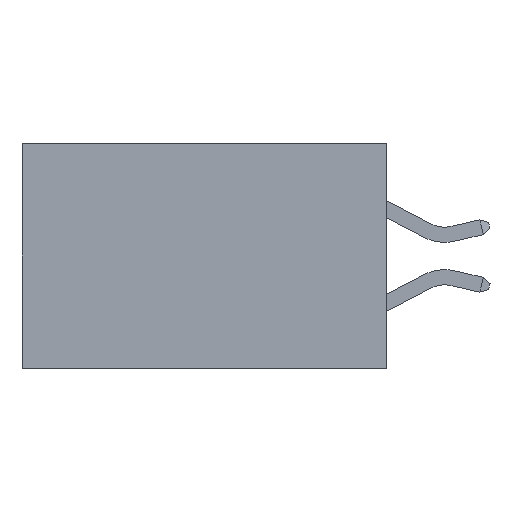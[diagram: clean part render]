
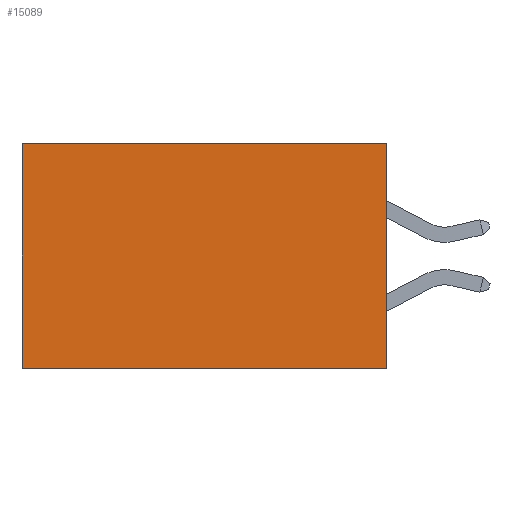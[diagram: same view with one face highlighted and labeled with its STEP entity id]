
A CAD part, left-side view. The second image highlights one B-rep face of the part: STEP entity #15089.
In plain terms, the highlighted planar face has unit normal (-1, 0, 0).
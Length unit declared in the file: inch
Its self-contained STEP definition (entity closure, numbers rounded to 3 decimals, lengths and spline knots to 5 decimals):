
#52 = VECTOR ( 'NONE', #13394, 39.37008 ) ;
#199 = LINE ( 'NONE', #14924, #10874 ) ;
#1112 = DIRECTION ( 'NONE',  ( 0., 0., -1. ) ) ;
#1361 = VECTOR ( 'NONE', #12651, 39.37008 ) ;
#1576 = CARTESIAN_POINT ( 'NONE',  ( 0.298, 0., 0. ) ) ;
#1749 = ORIENTED_EDGE ( 'NONE', *, *, #4311, .F. ) ;
#1804 = LINE ( 'NONE', #1576, #1361 ) ;
#1868 = EDGE_LOOP ( 'NONE', ( #5318, #17634, #1749, #15036 ) ) ;
#2588 = EDGE_CURVE ( 'NONE', #6344, #4546, #7381, .T. ) ;
#3395 = EDGE_CURVE ( 'NONE', #5895, #10210, #1804, .T. ) ;
#3590 = CARTESIAN_POINT ( 'NONE',  ( 0.298, 0., 0. ) ) ;
#3687 = LINE ( 'NONE', #9268, #52 ) ;
#3765 = CARTESIAN_POINT ( 'NONE',  ( 0.298, 0., 0. ) ) ;
#4311 = EDGE_CURVE ( 'NONE', #5895, #6344, #3687, .T. ) ;
#4328 = FACE_OUTER_BOUND ( 'NONE', #1868, .T. ) ;
#4546 = VERTEX_POINT ( 'NONE', #12288 ) ;
#5318 = ORIENTED_EDGE ( 'NONE', *, *, #7977, .T. ) ;
#5843 = CARTESIAN_POINT ( 'NONE',  ( 0.298, 0.6, 0. ) ) ;
#5895 = VERTEX_POINT ( 'NONE', #3590 ) ;
#6344 = VERTEX_POINT ( 'NONE', #8497 ) ;
#7381 = LINE ( 'NONE', #15487, #14379 ) ;
#7475 = DIRECTION ( 'NONE',  ( 0., 1., 0. ) ) ;
#7977 = EDGE_CURVE ( 'NONE', #10210, #4546, #199, .T. ) ;
#8098 = DIRECTION ( 'NONE',  ( 0., 0., -1. ) ) ;
#8497 = CARTESIAN_POINT ( 'NONE',  ( 0.298, 0., -0.37 ) ) ;
#9268 = CARTESIAN_POINT ( 'NONE',  ( 0.298, 0., 0. ) ) ;
#9335 = PLANE ( 'NONE',  #15754 ) ;
#10210 = VERTEX_POINT ( 'NONE', #5843 ) ;
#10874 = VECTOR ( 'NONE', #8098, 39.37008 ) ;
#12288 = CARTESIAN_POINT ( 'NONE',  ( 0.298, 0.6, -0.37 ) ) ;
#12651 = DIRECTION ( 'NONE',  ( 0., 1., 0. ) ) ;
#13394 = DIRECTION ( 'NONE',  ( 0., 0., -1. ) ) ;
#14379 = VECTOR ( 'NONE', #7475, 39.37008 ) ;
#14924 = CARTESIAN_POINT ( 'NONE',  ( 0.298, 0.6, 0. ) ) ;
#15036 = ORIENTED_EDGE ( 'NONE', *, *, #3395, .T. ) ;
#15089 = ADVANCED_FACE ( 'NONE', ( #4328 ), #9335, .F. ) ;
#15487 = CARTESIAN_POINT ( 'NONE',  ( 0.298, 0., -0.37 ) ) ;
#15754 = AXIS2_PLACEMENT_3D ( 'NONE', #3765, #17223, #1112 ) ;
#17223 = DIRECTION ( 'NONE',  ( 1., 0., 0. ) ) ;
#17634 = ORIENTED_EDGE ( 'NONE', *, *, #2588, .F. ) ;
